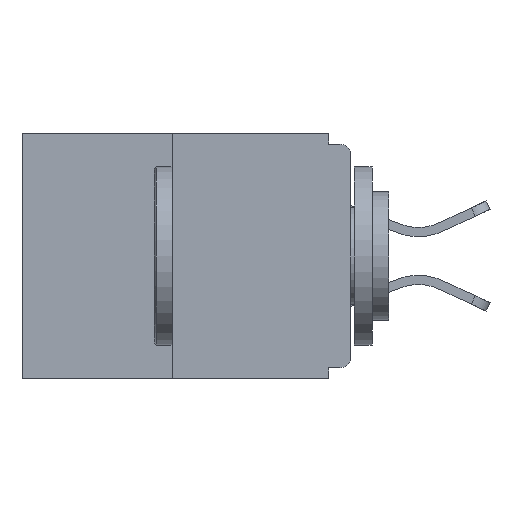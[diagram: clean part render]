
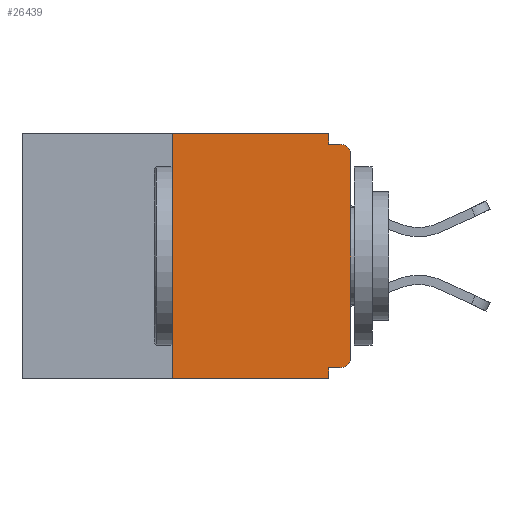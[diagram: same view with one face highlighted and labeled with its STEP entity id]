
A CAD part, left-side view. The second image highlights one B-rep face of the part: STEP entity #26439.
In plain terms, the highlighted planar face has unit normal (-1, 0, 0).
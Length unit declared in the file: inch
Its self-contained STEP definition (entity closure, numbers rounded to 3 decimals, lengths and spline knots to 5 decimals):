
#222 = DIRECTION ( 'NONE',  ( 0., -1., 0. ) ) ;
#248 = EDGE_LOOP ( 'NONE', ( #3311, #12591, #5266, #19999, #20973, #13206, #12808, #514, #16477, #18453 ) ) ;
#514 = ORIENTED_EDGE ( 'NONE', *, *, #4731, .T. ) ;
#545 = LINE ( 'NONE', #19199, #4464 ) ;
#737 = EDGE_CURVE ( 'NONE', #22779, #17729, #21529, .T. ) ;
#890 = CARTESIAN_POINT ( 'NONE',  ( 0., 0.031, 0. ) ) ;
#1212 = VECTOR ( 'NONE', #6940, 39.37008 ) ;
#1292 = EDGE_CURVE ( 'NONE', #17729, #3085, #6893, .T. ) ;
#1644 = DIRECTION ( 'NONE',  ( 0., 0., -1. ) ) ;
#1667 = DIRECTION ( 'NONE',  ( 0., -1., 0. ) ) ;
#1766 = EDGE_CURVE ( 'NONE', #27307, #18699, #18006, .T. ) ;
#2043 = CARTESIAN_POINT ( 'NONE',  ( 0., 0.46, 0. ) ) ;
#2210 = LINE ( 'NONE', #13718, #19704 ) ;
#2248 = DIRECTION ( 'NONE',  ( 0., 0., -1. ) ) ;
#2760 = DIRECTION ( 'NONE',  ( -1., 0., 0. ) ) ;
#2828 = CIRCLE ( 'NONE', #13631, 0.015 ) ;
#2899 = EDGE_CURVE ( 'NONE', #18863, #27307, #10800, .T. ) ;
#3085 = VERTEX_POINT ( 'NONE', #890 ) ;
#3311 = ORIENTED_EDGE ( 'NONE', *, *, #1292, .F. ) ;
#3337 = EDGE_CURVE ( 'NONE', #18863, #28164, #2210, .T. ) ;
#3890 = CARTESIAN_POINT ( 'NONE',  ( 0., 0.015, -0.328 ) ) ;
#4464 = VECTOR ( 'NONE', #12489, 39.37008 ) ;
#4731 = EDGE_CURVE ( 'NONE', #18699, #24995, #2828, .T. ) ;
#4858 = DIRECTION ( 'NONE',  ( 0., 0., -1. ) ) ;
#5266 = ORIENTED_EDGE ( 'NONE', *, *, #28859, .T. ) ;
#6029 = AXIS2_PLACEMENT_3D ( 'NONE', #2043, #9103, #2248 ) ;
#6631 = LINE ( 'NONE', #13408, #21995 ) ;
#6893 = LINE ( 'NONE', #16266, #23684 ) ;
#6940 = DIRECTION ( 'NONE',  ( 0., 0., 1. ) ) ;
#7272 = VERTEX_POINT ( 'NONE', #21452 ) ;
#7644 = EDGE_CURVE ( 'NONE', #28164, #24180, #545, .T. ) ;
#7979 = AXIS2_PLACEMENT_3D ( 'NONE', #27638, #27454, #9651 ) ;
#9103 = DIRECTION ( 'NONE',  ( 1., 0., 0. ) ) ;
#9651 = DIRECTION ( 'NONE',  ( 0., 0., -1. ) ) ;
#10800 = CIRCLE ( 'NONE', #7979, 0.015 ) ;
#10933 = CARTESIAN_POINT ( 'NONE',  ( 0., 0.031, -0.328 ) ) ;
#11017 = CARTESIAN_POINT ( 'NONE',  ( 0., 0.031, 0. ) ) ;
#12489 = DIRECTION ( 'NONE',  ( 0., 0., -1. ) ) ;
#12591 = ORIENTED_EDGE ( 'NONE', *, *, #737, .F. ) ;
#12808 = ORIENTED_EDGE ( 'NONE', *, *, #1766, .T. ) ;
#13206 = ORIENTED_EDGE ( 'NONE', *, *, #2899, .T. ) ;
#13408 = CARTESIAN_POINT ( 'NONE',  ( 0., 0.46, -0.343 ) ) ;
#13631 = AXIS2_PLACEMENT_3D ( 'NONE', #27457, #2760, #4858 ) ;
#13718 = CARTESIAN_POINT ( 'NONE',  ( 0., 0., -0.328 ) ) ;
#15296 = VECTOR ( 'NONE', #1667, 39.37008 ) ;
#15824 = PLANE ( 'NONE',  #6029 ) ;
#16266 = CARTESIAN_POINT ( 'NONE',  ( 0., 0.46, 0. ) ) ;
#16477 = ORIENTED_EDGE ( 'NONE', *, *, #23511, .F. ) ;
#17729 = VERTEX_POINT ( 'NONE', #24674 ) ;
#18006 = LINE ( 'NONE', #22838, #25111 ) ;
#18260 = CARTESIAN_POINT ( 'NONE',  ( 0., 0.015, -0.015 ) ) ;
#18453 = ORIENTED_EDGE ( 'NONE', *, *, #19486, .F. ) ;
#18650 = CARTESIAN_POINT ( 'NONE',  ( 0., 0., -0.313 ) ) ;
#18699 = VERTEX_POINT ( 'NONE', #23941 ) ;
#18863 = VERTEX_POINT ( 'NONE', #3890 ) ;
#19199 = CARTESIAN_POINT ( 'NONE',  ( 0., 0.031, -0.343 ) ) ;
#19486 = EDGE_CURVE ( 'NONE', #3085, #7272, #20188, .T. ) ;
#19704 = VECTOR ( 'NONE', #22575, 39.37008 ) ;
#19942 = CARTESIAN_POINT ( 'NONE',  ( 0., 0.25, 0. ) ) ;
#19999 = ORIENTED_EDGE ( 'NONE', *, *, #7644, .F. ) ;
#20188 = LINE ( 'NONE', #11017, #24117 ) ;
#20972 = CARTESIAN_POINT ( 'NONE',  ( 0., 0.25, -0.343 ) ) ;
#20973 = ORIENTED_EDGE ( 'NONE', *, *, #3337, .F. ) ;
#21343 = LINE ( 'NONE', #22014, #15296 ) ;
#21452 = CARTESIAN_POINT ( 'NONE',  ( 0., 0.031, -0.015 ) ) ;
#21529 = LINE ( 'NONE', #19942, #1212 ) ;
#21995 = VECTOR ( 'NONE', #27094, 39.37008 ) ;
#22014 = CARTESIAN_POINT ( 'NONE',  ( 0., 0., -0.015 ) ) ;
#22531 = DIRECTION ( 'NONE',  ( 0., 0., 1. ) ) ;
#22575 = DIRECTION ( 'NONE',  ( 0., 1., 0. ) ) ;
#22779 = VERTEX_POINT ( 'NONE', #20972 ) ;
#22838 = CARTESIAN_POINT ( 'NONE',  ( 0., 0., 0. ) ) ;
#23511 = EDGE_CURVE ( 'NONE', #7272, #24995, #21343, .T. ) ;
#23684 = VECTOR ( 'NONE', #222, 39.37008 ) ;
#23941 = CARTESIAN_POINT ( 'NONE',  ( 0., 0., -0.03 ) ) ;
#24117 = VECTOR ( 'NONE', #1644, 39.37008 ) ;
#24180 = VERTEX_POINT ( 'NONE', #26744 ) ;
#24674 = CARTESIAN_POINT ( 'NONE',  ( 0., 0.25, 0. ) ) ;
#24995 = VERTEX_POINT ( 'NONE', #18260 ) ;
#25111 = VECTOR ( 'NONE', #22531, 39.37008 ) ;
#26070 = FACE_OUTER_BOUND ( 'NONE', #248, .T. ) ;
#26439 = ADVANCED_FACE ( 'NONE', ( #26070 ), #15824, .F. ) ;
#26744 = CARTESIAN_POINT ( 'NONE',  ( 0., 0.031, -0.343 ) ) ;
#27094 = DIRECTION ( 'NONE',  ( 0., -1., 0. ) ) ;
#27307 = VERTEX_POINT ( 'NONE', #18650 ) ;
#27454 = DIRECTION ( 'NONE',  ( -1., 0., 0. ) ) ;
#27457 = CARTESIAN_POINT ( 'NONE',  ( 0., 0.015, -0.03 ) ) ;
#27638 = CARTESIAN_POINT ( 'NONE',  ( 0., 0.015, -0.313 ) ) ;
#28164 = VERTEX_POINT ( 'NONE', #10933 ) ;
#28859 = EDGE_CURVE ( 'NONE', #22779, #24180, #6631, .T. ) ;
